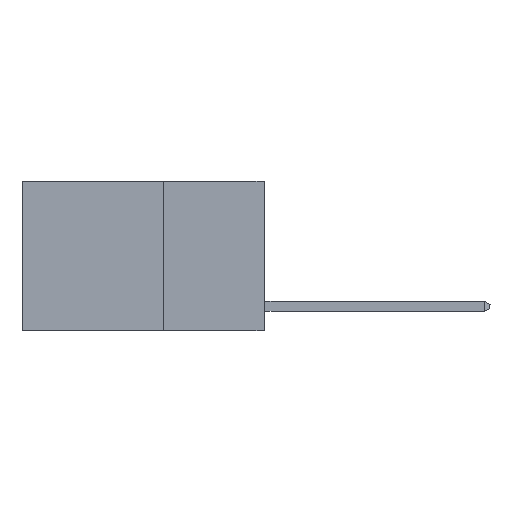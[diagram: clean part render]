
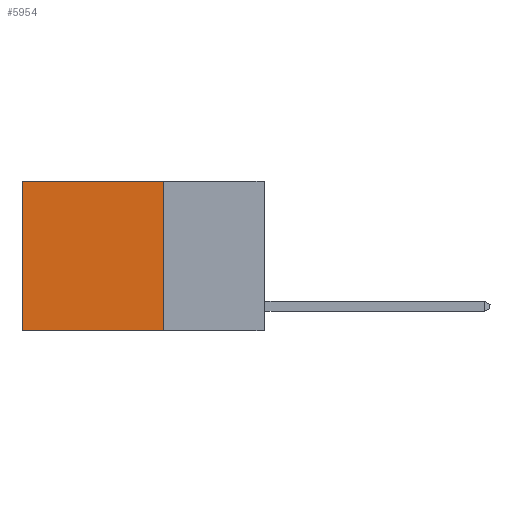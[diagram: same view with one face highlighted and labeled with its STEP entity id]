
A CAD part, left-side view. The second image highlights one B-rep face of the part: STEP entity #5954.
In plain terms, the highlighted planar face has unit normal (-1, 0, 0).
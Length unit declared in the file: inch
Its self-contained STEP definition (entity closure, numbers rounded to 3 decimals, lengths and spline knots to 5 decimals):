
#394 = EDGE_CURVE ( 'NONE', #9788, #4641, #8035, .T. ) ;
#1533 = DIRECTION ( 'NONE',  ( 0., 1., 0. ) ) ;
#1777 = CARTESIAN_POINT ( 'NONE',  ( 0.2625, 0.25, 0. ) ) ;
#1789 = DIRECTION ( 'NONE',  ( 0., 0., -1. ) ) ;
#1842 = LINE ( 'NONE', #11871, #6009 ) ;
#1925 = DIRECTION ( 'NONE',  ( 0., 1., 0. ) ) ;
#2017 = LINE ( 'NONE', #11621, #6781 ) ;
#2463 = CARTESIAN_POINT ( 'NONE',  ( 0.2625, 0.25, -0.37 ) ) ;
#2791 = CARTESIAN_POINT ( 'NONE',  ( 0.2625, 0.25, 0. ) ) ;
#4149 = AXIS2_PLACEMENT_3D ( 'NONE', #1777, #11861, #6557 ) ;
#4478 = CARTESIAN_POINT ( 'NONE',  ( 0.2625, 0.6, 0. ) ) ;
#4641 = VERTEX_POINT ( 'NONE', #9521 ) ;
#5495 = EDGE_CURVE ( 'NONE', #5964, #9788, #1842, .T. ) ;
#5624 = PLANE ( 'NONE',  #4149 ) ;
#5709 = FACE_OUTER_BOUND ( 'NONE', #7599, .T. ) ;
#5740 = CARTESIAN_POINT ( 'NONE',  ( 0.2625, 0.6, 0. ) ) ;
#5954 = ADVANCED_FACE ( 'NONE', ( #5709 ), #5624, .F. ) ;
#5964 = VERTEX_POINT ( 'NONE', #2791 ) ;
#6009 = VECTOR ( 'NONE', #1789, 39.37008 ) ;
#6356 = CARTESIAN_POINT ( 'NONE',  ( 0.2625, 0.25, -0.37 ) ) ;
#6557 = DIRECTION ( 'NONE',  ( 0., 0., -1. ) ) ;
#6781 = VECTOR ( 'NONE', #1533, 39.37008 ) ;
#7599 = EDGE_LOOP ( 'NONE', ( #8103, #8158, #8299, #8396 ) ) ;
#7606 = EDGE_CURVE ( 'NONE', #10252, #4641, #8939, .T. ) ;
#8035 = LINE ( 'NONE', #2463, #8308 ) ;
#8103 = ORIENTED_EDGE ( 'NONE', *, *, #7606, .T. ) ;
#8158 = ORIENTED_EDGE ( 'NONE', *, *, #394, .F. ) ;
#8299 = ORIENTED_EDGE ( 'NONE', *, *, #5495, .F. ) ;
#8308 = VECTOR ( 'NONE', #1925, 39.37008 ) ;
#8396 = ORIENTED_EDGE ( 'NONE', *, *, #9733, .T. ) ;
#8939 = LINE ( 'NONE', #4478, #10916 ) ;
#9521 = CARTESIAN_POINT ( 'NONE',  ( 0.2625, 0.6, -0.37 ) ) ;
#9733 = EDGE_CURVE ( 'NONE', #5964, #10252, #2017, .T. ) ;
#9788 = VERTEX_POINT ( 'NONE', #6356 ) ;
#9989 = DIRECTION ( 'NONE',  ( 0., 0., -1. ) ) ;
#10252 = VERTEX_POINT ( 'NONE', #5740 ) ;
#10916 = VECTOR ( 'NONE', #9989, 39.37008 ) ;
#11621 = CARTESIAN_POINT ( 'NONE',  ( 0.2625, 0.25, 0. ) ) ;
#11861 = DIRECTION ( 'NONE',  ( 1., 0., 0. ) ) ;
#11871 = CARTESIAN_POINT ( 'NONE',  ( 0.2625, 0.25, 0. ) ) ;
